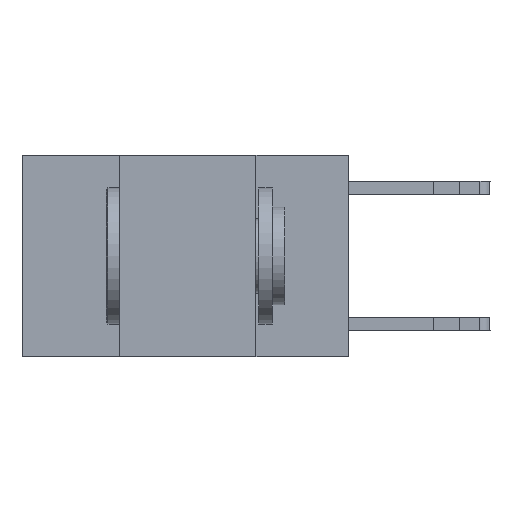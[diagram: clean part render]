
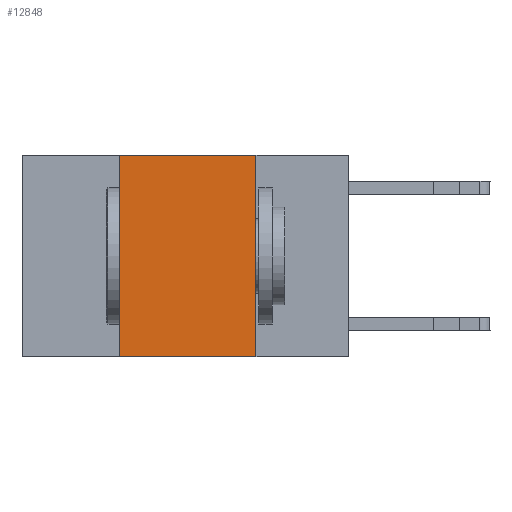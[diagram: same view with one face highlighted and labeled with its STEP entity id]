
A CAD part, left-side view. The second image highlights one B-rep face of the part: STEP entity #12848.
In plain terms, the highlighted planar face has unit normal (-1, 0, 0).
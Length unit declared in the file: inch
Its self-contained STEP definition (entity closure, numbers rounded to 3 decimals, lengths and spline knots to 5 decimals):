
#134 = VERTEX_POINT ( 'NONE', #8625 ) ;
#917 = CARTESIAN_POINT ( 'NONE',  ( 0., 0.17, 0. ) ) ;
#1031 = ORIENTED_EDGE ( 'NONE', *, *, #12974, .T. ) ;
#1062 = LINE ( 'NONE', #6261, #4250 ) ;
#1789 = VECTOR ( 'NONE', #7150, 39.37008 ) ;
#2305 = VECTOR ( 'NONE', #6999, 39.37008 ) ;
#2396 = ORIENTED_EDGE ( 'NONE', *, *, #12719, .F. ) ;
#3631 = CARTESIAN_POINT ( 'NONE',  ( 0., 0.6, 0. ) ) ;
#3675 = EDGE_CURVE ( 'NONE', #6709, #5218, #7202, .T. ) ;
#3876 = EDGE_CURVE ( 'NONE', #134, #6709, #11216, .T. ) ;
#4250 = VECTOR ( 'NONE', #7160, 39.37008 ) ;
#5218 = VERTEX_POINT ( 'NONE', #917 ) ;
#5847 = FACE_OUTER_BOUND ( 'NONE', #13328, .T. ) ;
#6261 = CARTESIAN_POINT ( 'NONE',  ( 0., 0.6, -0.37 ) ) ;
#6456 = AXIS2_PLACEMENT_3D ( 'NONE', #3631, #9093, #13254 ) ;
#6709 = VERTEX_POINT ( 'NONE', #8679 ) ;
#6764 = LINE ( 'NONE', #8575, #7755 ) ;
#6787 = ORIENTED_EDGE ( 'NONE', *, *, #3876, .F. ) ;
#6999 = DIRECTION ( 'NONE',  ( 0., -1., 0. ) ) ;
#7027 = PLANE ( 'NONE',  #6456 ) ;
#7150 = DIRECTION ( 'NONE',  ( 0., 0., 1. ) ) ;
#7160 = DIRECTION ( 'NONE',  ( 0., -1., 0. ) ) ;
#7202 = LINE ( 'NONE', #11333, #2305 ) ;
#7509 = DIRECTION ( 'NONE',  ( 0., 0., -1. ) ) ;
#7755 = VECTOR ( 'NONE', #7509, 39.37008 ) ;
#8098 = CARTESIAN_POINT ( 'NONE',  ( 0., 0.17, -0.37 ) ) ;
#8575 = CARTESIAN_POINT ( 'NONE',  ( 0., 0.17, 0. ) ) ;
#8625 = CARTESIAN_POINT ( 'NONE',  ( 0., 0.42, -0.37 ) ) ;
#8635 = ORIENTED_EDGE ( 'NONE', *, *, #3675, .F. ) ;
#8679 = CARTESIAN_POINT ( 'NONE',  ( 0., 0.42, 0. ) ) ;
#9093 = DIRECTION ( 'NONE',  ( 1., 0., 0. ) ) ;
#9287 = CARTESIAN_POINT ( 'NONE',  ( 0., 0.42, 0. ) ) ;
#11216 = LINE ( 'NONE', #9287, #1789 ) ;
#11333 = CARTESIAN_POINT ( 'NONE',  ( 0., 0.6, 0. ) ) ;
#12719 = EDGE_CURVE ( 'NONE', #5218, #12791, #6764, .T. ) ;
#12791 = VERTEX_POINT ( 'NONE', #8098 ) ;
#12848 = ADVANCED_FACE ( 'NONE', ( #5847 ), #7027, .F. ) ;
#12974 = EDGE_CURVE ( 'NONE', #134, #12791, #1062, .T. ) ;
#13254 = DIRECTION ( 'NONE',  ( 0., 0., -1. ) ) ;
#13328 = EDGE_LOOP ( 'NONE', ( #2396, #8635, #6787, #1031 ) ) ;
